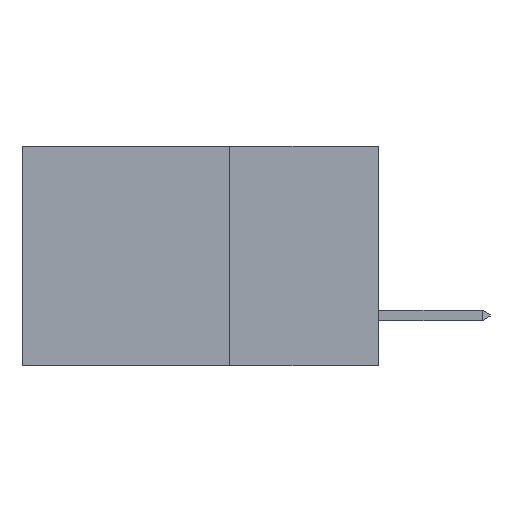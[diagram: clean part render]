
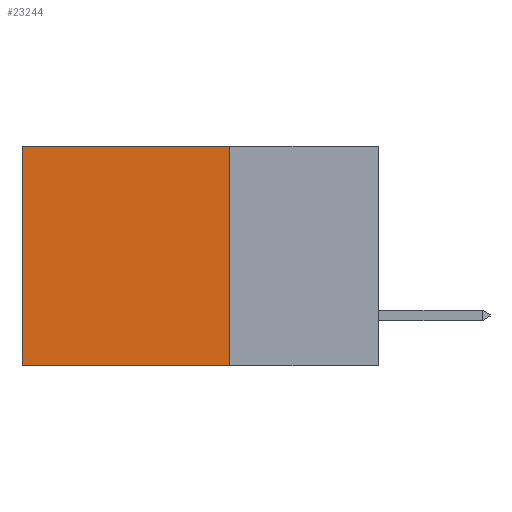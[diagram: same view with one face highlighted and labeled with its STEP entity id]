
A CAD part, left-side view. The second image highlights one B-rep face of the part: STEP entity #23244.
In plain terms, the highlighted planar face has unit normal (-1, 0, 0).
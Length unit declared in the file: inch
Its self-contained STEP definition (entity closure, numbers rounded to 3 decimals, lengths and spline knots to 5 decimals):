
#301 = PLANE ( 'NONE',  #19142 ) ;
#927 = VECTOR ( 'NONE', #29096, 39.37008 ) ;
#1057 = CARTESIAN_POINT ( 'NONE',  ( 0.298, 0.25, -0.37 ) ) ;
#1341 = VECTOR ( 'NONE', #12069, 39.37008 ) ;
#1401 = VECTOR ( 'NONE', #4917, 39.37008 ) ;
#2178 = LINE ( 'NONE', #12386, #1401 ) ;
#2802 = CARTESIAN_POINT ( 'NONE',  ( 0.298, 0.25, 0. ) ) ;
#4005 = EDGE_CURVE ( 'NONE', #25784, #20268, #26880, .T. ) ;
#4886 = ORIENTED_EDGE ( 'NONE', *, *, #19838, .T. ) ;
#4917 = DIRECTION ( 'NONE',  ( 0., 0., -1. ) ) ;
#5282 = DIRECTION ( 'NONE',  ( 1., 0., 0. ) ) ;
#5543 = EDGE_LOOP ( 'NONE', ( #16164, #5742, #25187, #4886 ) ) ;
#5742 = ORIENTED_EDGE ( 'NONE', *, *, #4005, .F. ) ;
#6926 = CARTESIAN_POINT ( 'NONE',  ( 0.298, 0.25, 0. ) ) ;
#7298 = VERTEX_POINT ( 'NONE', #17260 ) ;
#7825 = CARTESIAN_POINT ( 'NONE',  ( 0.298, 0.25, 0. ) ) ;
#8154 = VERTEX_POINT ( 'NONE', #20377 ) ;
#12069 = DIRECTION ( 'NONE',  ( 0., 1., 0. ) ) ;
#12386 = CARTESIAN_POINT ( 'NONE',  ( 0.298, 0.6, 0. ) ) ;
#14193 = EDGE_CURVE ( 'NONE', #8154, #25784, #16946, .T. ) ;
#15927 = CARTESIAN_POINT ( 'NONE',  ( 0.298, 0.6, -0.37 ) ) ;
#16164 = ORIENTED_EDGE ( 'NONE', *, *, #30433, .T. ) ;
#16946 = LINE ( 'NONE', #7825, #29930 ) ;
#17260 = CARTESIAN_POINT ( 'NONE',  ( 0.298, 0.6, 0. ) ) ;
#17787 = FACE_OUTER_BOUND ( 'NONE', #5543, .T. ) ;
#18471 = CARTESIAN_POINT ( 'NONE',  ( 0.298, 0.25, -0.37 ) ) ;
#19142 = AXIS2_PLACEMENT_3D ( 'NONE', #2802, #5282, #22679 ) ;
#19838 = EDGE_CURVE ( 'NONE', #8154, #7298, #20768, .T. ) ;
#20268 = VERTEX_POINT ( 'NONE', #15927 ) ;
#20377 = CARTESIAN_POINT ( 'NONE',  ( 0.298, 0.25, 0. ) ) ;
#20768 = LINE ( 'NONE', #6926, #927 ) ;
#22679 = DIRECTION ( 'NONE',  ( 0., 0., -1. ) ) ;
#23244 = ADVANCED_FACE ( 'NONE', ( #17787 ), #301, .F. ) ;
#25126 = DIRECTION ( 'NONE',  ( 0., 0., -1. ) ) ;
#25187 = ORIENTED_EDGE ( 'NONE', *, *, #14193, .F. ) ;
#25784 = VERTEX_POINT ( 'NONE', #18471 ) ;
#26880 = LINE ( 'NONE', #1057, #1341 ) ;
#29096 = DIRECTION ( 'NONE',  ( 0., 1., 0. ) ) ;
#29930 = VECTOR ( 'NONE', #25126, 39.37008 ) ;
#30433 = EDGE_CURVE ( 'NONE', #7298, #20268, #2178, .T. ) ;
